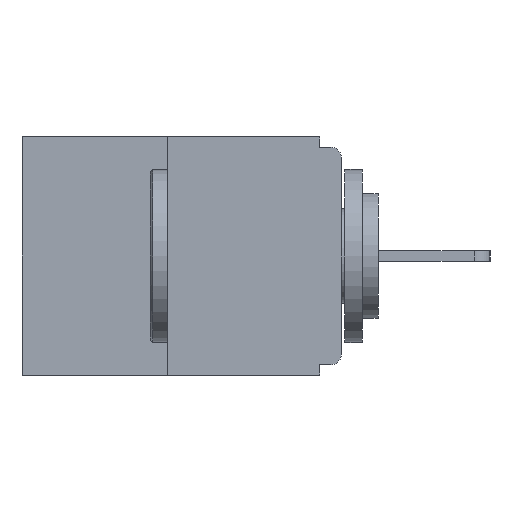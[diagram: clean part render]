
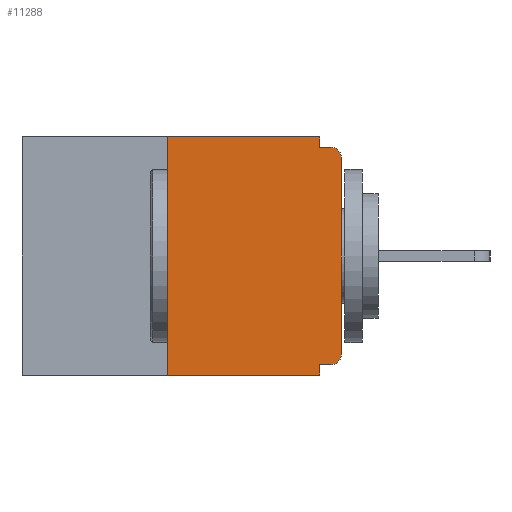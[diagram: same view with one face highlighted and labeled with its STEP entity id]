
A CAD part, left-side view. The second image highlights one B-rep face of the part: STEP entity #11288.
In plain terms, the highlighted planar face has unit normal (-1, 0, 0).
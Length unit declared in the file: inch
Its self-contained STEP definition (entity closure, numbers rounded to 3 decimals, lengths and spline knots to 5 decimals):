
#38 = CARTESIAN_POINT ( 'NONE',  ( 0., 0.015, -0.015 ) ) ;
#352 = CARTESIAN_POINT ( 'NONE',  ( 0., 0.031, 0. ) ) ;
#478 = VECTOR ( 'NONE', #10604, 39.37008 ) ;
#635 = ORIENTED_EDGE ( 'NONE', *, *, #5524, .F. ) ;
#864 = EDGE_CURVE ( 'NONE', #10652, #3724, #6895, .T. ) ;
#922 = CARTESIAN_POINT ( 'NONE',  ( 0., 0.25, 0. ) ) ;
#1824 = VERTEX_POINT ( 'NONE', #38 ) ;
#1993 = AXIS2_PLACEMENT_3D ( 'NONE', #10670, #7891, #10580 ) ;
#2228 = PLANE ( 'NONE',  #17159 ) ;
#2251 = VECTOR ( 'NONE', #14865, 39.37008 ) ;
#2318 = ORIENTED_EDGE ( 'NONE', *, *, #12697, .F. ) ;
#2463 = CARTESIAN_POINT ( 'NONE',  ( 0., 0.46, 0. ) ) ;
#2543 = EDGE_CURVE ( 'NONE', #8691, #4243, #17435, .T. ) ;
#3344 = DIRECTION ( 'NONE',  ( 0., 0., -1. ) ) ;
#3510 = CARTESIAN_POINT ( 'NONE',  ( 0., 0.031, 0. ) ) ;
#3532 = DIRECTION ( 'NONE',  ( 0., -1., 0. ) ) ;
#3556 = CARTESIAN_POINT ( 'NONE',  ( 0., 0.46, 0. ) ) ;
#3582 = EDGE_CURVE ( 'NONE', #17490, #4144, #7825, .T. ) ;
#3689 = CIRCLE ( 'NONE', #1993, 0.015 ) ;
#3724 = VERTEX_POINT ( 'NONE', #9828 ) ;
#3898 = VERTEX_POINT ( 'NONE', #12803 ) ;
#3996 = DIRECTION ( 'NONE',  ( -1., 0., 0. ) ) ;
#4123 = CARTESIAN_POINT ( 'NONE',  ( 0., 0., 0. ) ) ;
#4144 = VERTEX_POINT ( 'NONE', #9664 ) ;
#4243 = VERTEX_POINT ( 'NONE', #352 ) ;
#4272 = ORIENTED_EDGE ( 'NONE', *, *, #16231, .F. ) ;
#4976 = CARTESIAN_POINT ( 'NONE',  ( 0., 0., -0.015 ) ) ;
#5162 = DIRECTION ( 'NONE',  ( 0., 0., -1. ) ) ;
#5208 = CARTESIAN_POINT ( 'NONE',  ( 0., 0., -0.313 ) ) ;
#5336 = CARTESIAN_POINT ( 'NONE',  ( 0., 0.015, -0.03 ) ) ;
#5514 = VECTOR ( 'NONE', #3344, 39.37008 ) ;
#5524 = EDGE_CURVE ( 'NONE', #3898, #1824, #13054, .T. ) ;
#5575 = CARTESIAN_POINT ( 'NONE',  ( 0., 0.015, -0.328 ) ) ;
#5735 = VERTEX_POINT ( 'NONE', #16194 ) ;
#5942 = LINE ( 'NONE', #16901, #8751 ) ;
#6647 = ORIENTED_EDGE ( 'NONE', *, *, #2543, .F. ) ;
#6895 = LINE ( 'NONE', #4123, #9522 ) ;
#7101 = ORIENTED_EDGE ( 'NONE', *, *, #7801, .F. ) ;
#7801 = EDGE_CURVE ( 'NONE', #17490, #8691, #14546, .T. ) ;
#7816 = DIRECTION ( 'NONE',  ( 0., 0., 1. ) ) ;
#7825 = LINE ( 'NONE', #15894, #8397 ) ;
#7891 = DIRECTION ( 'NONE',  ( -1., 0., 0. ) ) ;
#7963 = CARTESIAN_POINT ( 'NONE',  ( 0., 0., -0.328 ) ) ;
#8397 = VECTOR ( 'NONE', #3532, 39.37008 ) ;
#8551 = EDGE_CURVE ( 'NONE', #3724, #1824, #9695, .T. ) ;
#8633 = LINE ( 'NONE', #3510, #5514 ) ;
#8691 = VERTEX_POINT ( 'NONE', #15385 ) ;
#8751 = VECTOR ( 'NONE', #9813, 39.37008 ) ;
#8881 = ORIENTED_EDGE ( 'NONE', *, *, #864, .T. ) ;
#9183 = ORIENTED_EDGE ( 'NONE', *, *, #8551, .T. ) ;
#9522 = VECTOR ( 'NONE', #12891, 39.37008 ) ;
#9664 = CARTESIAN_POINT ( 'NONE',  ( 0., 0.031, -0.343 ) ) ;
#9695 = CIRCLE ( 'NONE', #17709, 0.015 ) ;
#9747 = EDGE_CURVE ( 'NONE', #10333, #5735, #10646, .T. ) ;
#9813 = DIRECTION ( 'NONE',  ( 0., 0., -1. ) ) ;
#9828 = CARTESIAN_POINT ( 'NONE',  ( 0., 0., -0.03 ) ) ;
#10333 = VERTEX_POINT ( 'NONE', #5575 ) ;
#10543 = DIRECTION ( 'NONE',  ( 1., 0., 0. ) ) ;
#10580 = DIRECTION ( 'NONE',  ( 0., 0., -1. ) ) ;
#10604 = DIRECTION ( 'NONE',  ( 0., -1., 0. ) ) ;
#10646 = LINE ( 'NONE', #7963, #2251 ) ;
#10652 = VERTEX_POINT ( 'NONE', #5208 ) ;
#10670 = CARTESIAN_POINT ( 'NONE',  ( 0., 0.015, -0.313 ) ) ;
#10995 = EDGE_CURVE ( 'NONE', #10333, #10652, #3689, .T. ) ;
#11117 = EDGE_LOOP ( 'NONE', ( #6647, #7101, #16707, #4272, #17623, #16324, #8881, #9183, #635, #2318 ) ) ;
#11288 = ADVANCED_FACE ( 'NONE', ( #11516 ), #2228, .F. ) ;
#11516 = FACE_OUTER_BOUND ( 'NONE', #11117, .T. ) ;
#12697 = EDGE_CURVE ( 'NONE', #4243, #3898, #8633, .T. ) ;
#12803 = CARTESIAN_POINT ( 'NONE',  ( 0., 0.031, -0.015 ) ) ;
#12891 = DIRECTION ( 'NONE',  ( 0., 0., 1. ) ) ;
#13054 = LINE ( 'NONE', #4976, #17090 ) ;
#14312 = DIRECTION ( 'NONE',  ( 0., 0., -1. ) ) ;
#14495 = DIRECTION ( 'NONE',  ( 0., -1., 0. ) ) ;
#14546 = LINE ( 'NONE', #922, #15092 ) ;
#14781 = CARTESIAN_POINT ( 'NONE',  ( 0., 0.25, -0.343 ) ) ;
#14865 = DIRECTION ( 'NONE',  ( 0., 1., 0. ) ) ;
#15092 = VECTOR ( 'NONE', #7816, 39.37008 ) ;
#15385 = CARTESIAN_POINT ( 'NONE',  ( 0., 0.25, 0. ) ) ;
#15894 = CARTESIAN_POINT ( 'NONE',  ( 0., 0.46, -0.343 ) ) ;
#16194 = CARTESIAN_POINT ( 'NONE',  ( 0., 0.031, -0.328 ) ) ;
#16231 = EDGE_CURVE ( 'NONE', #5735, #4144, #5942, .T. ) ;
#16324 = ORIENTED_EDGE ( 'NONE', *, *, #10995, .T. ) ;
#16707 = ORIENTED_EDGE ( 'NONE', *, *, #3582, .T. ) ;
#16901 = CARTESIAN_POINT ( 'NONE',  ( 0., 0.031, -0.343 ) ) ;
#17090 = VECTOR ( 'NONE', #14495, 39.37008 ) ;
#17159 = AXIS2_PLACEMENT_3D ( 'NONE', #3556, #10543, #14312 ) ;
#17435 = LINE ( 'NONE', #2463, #478 ) ;
#17490 = VERTEX_POINT ( 'NONE', #14781 ) ;
#17623 = ORIENTED_EDGE ( 'NONE', *, *, #9747, .F. ) ;
#17709 = AXIS2_PLACEMENT_3D ( 'NONE', #5336, #3996, #5162 ) ;
